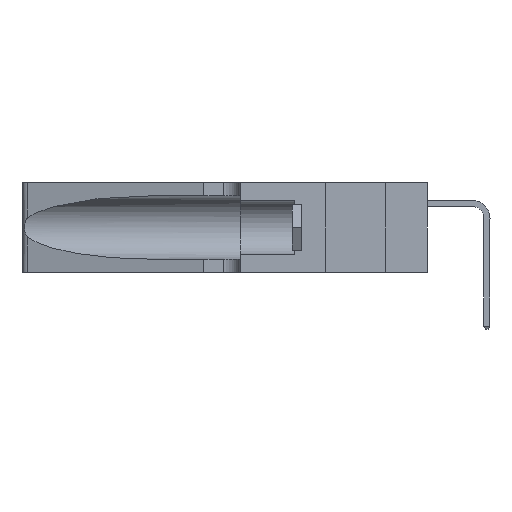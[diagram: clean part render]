
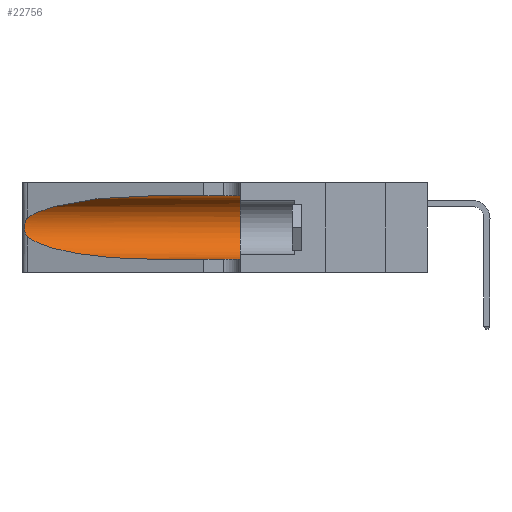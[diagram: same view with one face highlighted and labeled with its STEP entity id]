
A CAD part, left-side view. The second image highlights one B-rep face of the part: STEP entity #22756.
In plain terms, the highlighted cylindrical face has radius 3.308 mm (diameter 6.617 mm), a partial arc.
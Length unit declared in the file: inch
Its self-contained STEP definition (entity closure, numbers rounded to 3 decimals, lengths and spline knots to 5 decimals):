
#154 = DIRECTION ( 'NONE',  ( 0., 0., 1. ) ) ;
#165 = VERTEX_POINT ( 'NONE', #17315 ) ;
#1003 = CARTESIAN_POINT ( 'NONE',  ( 0.26017, 1.23833, 0.17102 ) ) ;
#1459 = DIRECTION ( 'NONE',  ( 0., -1., 0. ) ) ;
#2438 = ORIENTED_EDGE ( 'NONE', *, *, #10993, .T. ) ;
#2584 = CARTESIAN_POINT ( 'NONE',  ( 0.1305, 1.61858, 0.31525 ) ) ;
#2811 = ORIENTED_EDGE ( 'NONE', *, *, #13666, .T. ) ;
#2895 = CARTESIAN_POINT ( 'NONE',  ( 0.25487, 1.22718, 0.22369 ) ) ;
#3468 = FACE_OUTER_BOUND ( 'NONE', #19921, .T. ) ;
#3479 = CARTESIAN_POINT ( 'NONE',  ( 0.25789, 1.23486, 0.15765 ) ) ;
#5029 = CARTESIAN_POINT ( 'NONE',  ( 0.1305, 0.35, 0.31525 ) ) ;
#5228 = VERTEX_POINT ( 'NONE', #27650 ) ;
#5387 = CARTESIAN_POINT ( 'NONE',  ( 0.25487, 1.22718, 0.14631 ) ) ;
#5928 = CARTESIAN_POINT ( 'NONE',  ( 0.25555, 1.22993, 0.14849 ) ) ;
#7200 = ORIENTED_EDGE ( 'NONE', *, *, #9908, .T. ) ;
#7849 = CARTESIAN_POINT ( 'NONE',  ( 0.18966, 0.96281, 0.05475 ) ) ;
#8714 = EDGE_CURVE ( 'NONE', #14535, #5228, #18836, .T. ) ;
#8924 = ORIENTED_EDGE ( 'NONE', *, *, #8714, .F. ) ;
#9803 = AXIS2_PLACEMENT_3D ( 'NONE', #23104, #30146, #16045 ) ;
#9817 = CARTESIAN_POINT ( 'NONE',  ( 0.1305, 0.72297, 0.31525 ) ) ;
#9908 = EDGE_CURVE ( 'NONE', #29970, #165, #15798, .T. ) ;
#10099 = CARTESIAN_POINT ( 'NONE',  ( 0.18966, 0.96281, 0.31525 ) ) ;
#10658 = CARTESIAN_POINT ( 'NONE',  ( 0.25787, 1.23484, 0.2124 ) ) ;
#10993 = EDGE_CURVE ( 'NONE', #165, #26901, #21345, .T. ) ;
#12730 = EDGE_CURVE ( 'NONE', #26901, #20990, #26818, .T. ) ;
#12925 = CARTESIAN_POINT ( 'NONE',  ( 0.25555, 1.22994, 0.2215 ) ) ;
#13024 = CARTESIAN_POINT ( 'NONE',  ( 0.26018, 1.23835, 0.19895 ) ) ;
#13261 = VECTOR ( 'NONE', #19400, 39.37008 ) ;
#13666 = EDGE_CURVE ( 'NONE', #20990, #5228, #23145, .T. ) ;
#14015 = LINE ( 'NONE', #2584, #13261 ) ;
#14535 = VERTEX_POINT ( 'NONE', #5029 ) ;
#14609 = DIRECTION ( 'NONE',  ( 0., 1., 0. ) ) ;
#14908 = CARTESIAN_POINT ( 'NONE',  ( 0.2373, 1.15595, 0.08982 ) ) ;
#15427 = CARTESIAN_POINT ( 'NONE',  ( 0.26075, 1.23896, 0.178 ) ) ;
#15501 = ORIENTED_EDGE ( 'NONE', *, *, #25463, .F. ) ;
#15798 =( BOUNDED_CURVE ( )  B_SPLINE_CURVE ( 3, ( #26689, #10099, #17286, #2895 ),
 .UNSPECIFIED., .F., .T. ) 
 B_SPLINE_CURVE_WITH_KNOTS ( ( 4, 4 ),
 ( 1.5708, 2.84003 ),
 .UNSPECIFIED. ) 
 CURVE ( )  GEOMETRIC_REPRESENTATION_ITEM ( )  RATIONAL_B_SPLINE_CURVE ( ( 1., 0.87, 0.87, 1. ) ) 
 REPRESENTATION_ITEM ( '' )  );
#16045 = DIRECTION ( 'NONE',  ( 0., 0., -1. ) ) ;
#16848 = VECTOR ( 'NONE', #1459, 39.37008 ) ;
#17286 = CARTESIAN_POINT ( 'NONE',  ( 0.2373, 1.15595, 0.28018 ) ) ;
#17315 = CARTESIAN_POINT ( 'NONE',  ( 0.25487, 1.22718, 0.22369 ) ) ;
#17661 = CARTESIAN_POINT ( 'NONE',  ( 0.25487, 1.22718, 0.22369 ) ) ;
#17864 = CARTESIAN_POINT ( 'NONE',  ( 0.25856, 1.23593, 0.16098 ) ) ;
#18491 = ORIENTED_EDGE ( 'NONE', *, *, #12730, .T. ) ;
#18836 = CIRCLE ( 'NONE', #19535, 0.13025 ) ;
#19400 = DIRECTION ( 'NONE',  ( 0., -1., 0. ) ) ;
#19535 = AXIS2_PLACEMENT_3D ( 'NONE', #28778, #14609, #154 ) ;
#19921 = EDGE_LOOP ( 'NONE', ( #7200, #2438, #18491, #2811, #8924, #15501 ) ) ;
#19922 = CARTESIAN_POINT ( 'NONE',  ( 0.1305, 0.72297, 0.05475 ) ) ;
#20252 = CARTESIAN_POINT ( 'NONE',  ( 0.25639, 1.23186, 0.15144 ) ) ;
#20990 = VERTEX_POINT ( 'NONE', #19922 ) ;
#21073 = CYLINDRICAL_SURFACE ( 'NONE', #9803, 0.13025 ) ;
#21345 = B_SPLINE_CURVE_WITH_KNOTS ( 'NONE', 3,
 ( #17661, #12925, #24894, #10658, #27239, #13024, #29574, #15427, #1003, #17864, #3479, #20252, #5928, #22606 ),
 .UNSPECIFIED., .F., .F.,
 ( 4, 2, 2, 2, 2, 2, 4 ),
 ( 0., 0.00027, 0.00053, 0.00107, 0.0016, 0.00187, 0.00214 ),
 .UNSPECIFIED. ) ;
#22606 = CARTESIAN_POINT ( 'NONE',  ( 0.25487, 1.22718, 0.14631 ) ) ;
#22756 = ADVANCED_FACE ( 'NONE', ( #3468 ), #21073, .F. ) ;
#22943 = CARTESIAN_POINT ( 'NONE',  ( 0.1305, 1.61858, 0.05475 ) ) ;
#23104 = CARTESIAN_POINT ( 'NONE',  ( 0.1305, 1.61858, 0.185 ) ) ;
#23145 = LINE ( 'NONE', #22943, #16848 ) ;
#24484 = CARTESIAN_POINT ( 'NONE',  ( 0.1305, 0.72297, 0.05475 ) ) ;
#24793 = CARTESIAN_POINT ( 'NONE',  ( 0.25487, 1.22718, 0.14631 ) ) ;
#24894 = CARTESIAN_POINT ( 'NONE',  ( 0.25639, 1.23184, 0.21858 ) ) ;
#25463 = EDGE_CURVE ( 'NONE', #29970, #14535, #14015, .T. ) ;
#26689 = CARTESIAN_POINT ( 'NONE',  ( 0.1305, 0.72297, 0.31525 ) ) ;
#26818 =( BOUNDED_CURVE ( )  B_SPLINE_CURVE ( 3, ( #5387, #14908, #7849, #24484 ),
 .UNSPECIFIED., .F., .T. ) 
 B_SPLINE_CURVE_WITH_KNOTS ( ( 4, 4 ),
 ( 3.44316, 4.71239 ),
 .UNSPECIFIED. ) 
 CURVE ( )  GEOMETRIC_REPRESENTATION_ITEM ( )  RATIONAL_B_SPLINE_CURVE ( ( 1., 0.87, 0.87, 1. ) ) 
 REPRESENTATION_ITEM ( '' )  );
#26901 = VERTEX_POINT ( 'NONE', #24793 ) ;
#27239 = CARTESIAN_POINT ( 'NONE',  ( 0.25854, 1.2359, 0.20912 ) ) ;
#27650 = CARTESIAN_POINT ( 'NONE',  ( 0.1305, 0.35, 0.05475 ) ) ;
#28778 = CARTESIAN_POINT ( 'NONE',  ( 0.1305, 0.35, 0.185 ) ) ;
#29574 = CARTESIAN_POINT ( 'NONE',  ( 0.26075, 1.23896, 0.19203 ) ) ;
#29970 = VERTEX_POINT ( 'NONE', #9817 ) ;
#30146 = DIRECTION ( 'NONE',  ( 0., -1., 0. ) ) ;
